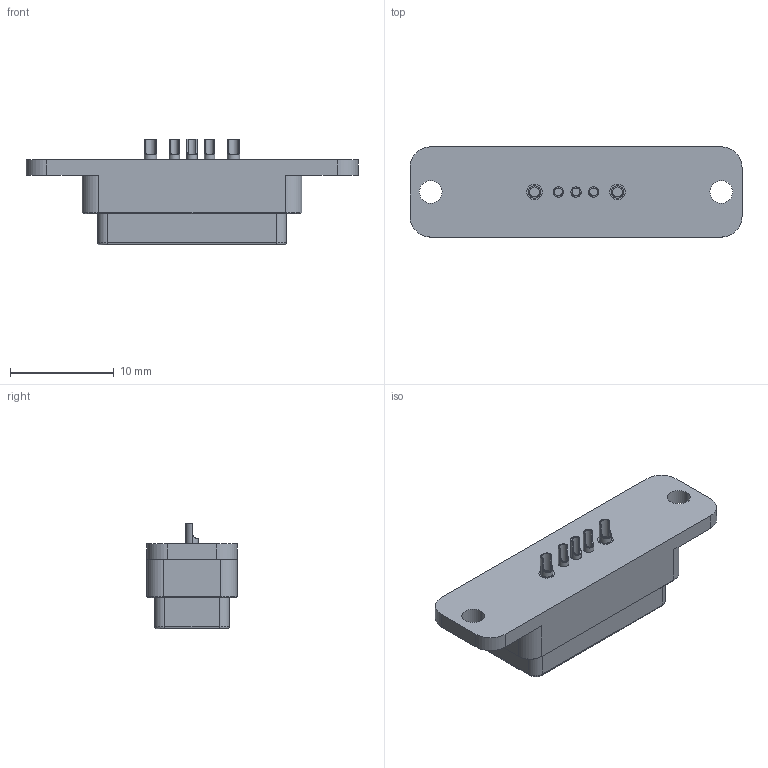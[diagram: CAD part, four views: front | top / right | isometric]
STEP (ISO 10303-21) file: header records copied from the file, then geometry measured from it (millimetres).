
FILE_DESCRIPTION (( 'STEP AP203' ), '1' );
FILE_NAME ('685K0551450113E.STEP', '2023-05-03T12:08:45', ( 'Magnum' ), ( '' ), 'SwSTEP 2.0', 'SolidWorks 2020', '' );
FILE_SCHEMA (( 'CONFIG_CONTROL_DESIGN' ));
Length unit declared in the file: millimetre
Products named in the file (1): 685K0551450113E
Bounding box: 32 x 8.7 x 10.2 mm (x, y, z)
Volume: 1396.6 mm3; surface area: 1163.8 mm2
Topology: 3 solids, 5 shells, 215 faces, 513 edges, 323 vertices
Faces by surface type: cylinder 87, plane 76, torus 24, bspline 24, cone 4
Entity records: 7943 total; most frequent: CARTESIAN_POINT 2841, DIRECTION 1076, ORIENTED_EDGE 1026, EDGE_CURVE 513, AXIS2_PLACEMENT_3D 418, VERTEX_POINT 323, EDGE_LOOP 242, LINE 240
